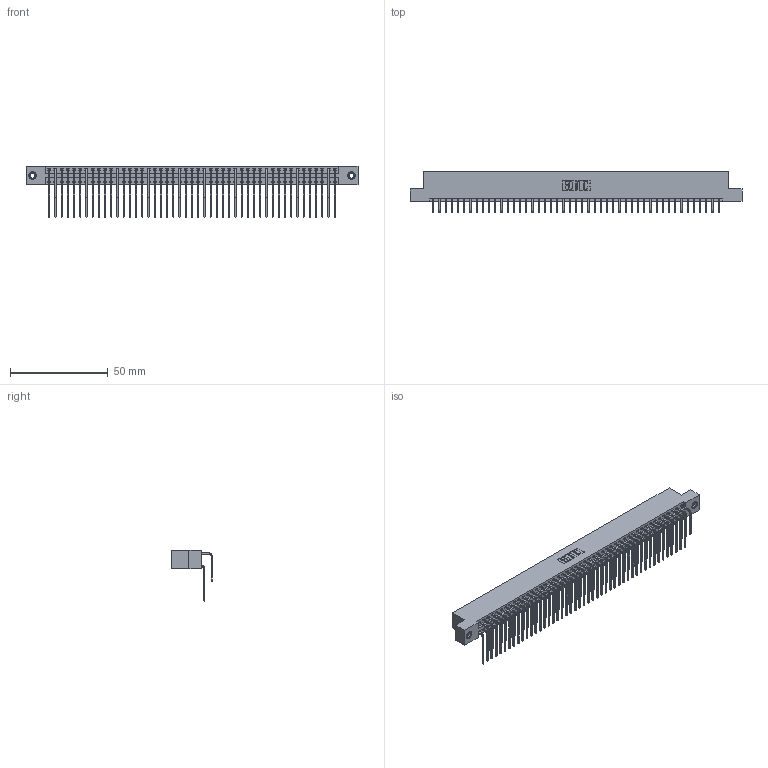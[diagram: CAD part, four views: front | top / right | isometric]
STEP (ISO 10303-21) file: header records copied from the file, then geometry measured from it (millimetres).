
FILE_DESCRIPTION (( 'STEP AP203' ), '1' );
FILE_NAME ('396-094-559-207.STEP', '2018-09-13T11:54:56', ( '' ), ( '' ), 'SwSTEP 2.0', 'SolidWorks 2016', '' );
FILE_SCHEMA (( 'CONFIG_CONTROL_DESIGN' ));
Length unit declared in the file: inch
Products named in the file (5): 345-292-001_559 Tail - 2; 345-250-001_345-250-005-103; 396-094-559-207; 346 Part_Flush Mounting Lugs - 0.156 Dia-TI; 345-292-001_558 559 Tail - 1
Assembly tree (97 placements, depth 2):
  396-094-559-207
    346 Part_Flush Mounting Lugs - 0.156 Dia-TI
    345-292-001_558 559 Tail - 1  x47
    345-292-001_559 Tail - 2  x47
    345-250-001_345-250-005-103  x2
Bounding box: 169.8 x 20.89 x 26.16 mm (x, y, z)
Volume: 17125.1 mm3; surface area: 26253.3 mm2
Topology: 97 solids, 97 shells, 5258 faces, 15599 edges, 10266 vertices
Faces by surface type: plane 3586, cylinder 1656, cone 12, torus 4
Entity records: 32970 total; most frequent: CARTESIAN_POINT 5462, ORIENTED_EDGE 5338, DIRECTION 4863, EDGE_CURVE 2669, VECTOR 2289, LINE 2289, VERTEX_POINT 1772, AXIS2_PLACEMENT_3D 1287
